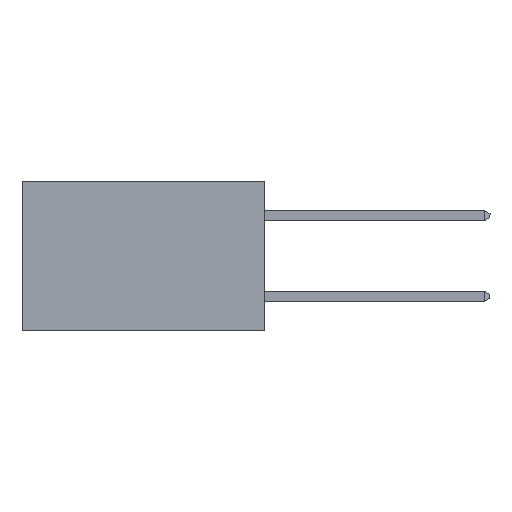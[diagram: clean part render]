
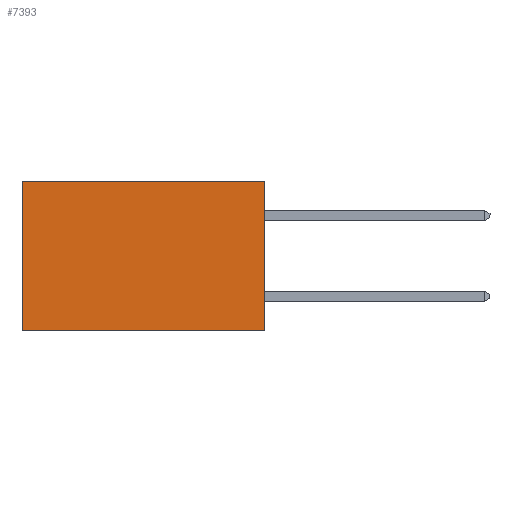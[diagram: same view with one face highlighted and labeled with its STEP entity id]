
A CAD part, left-side view. The second image highlights one B-rep face of the part: STEP entity #7393.
In plain terms, the highlighted planar face has unit normal (-1, 0, 0).
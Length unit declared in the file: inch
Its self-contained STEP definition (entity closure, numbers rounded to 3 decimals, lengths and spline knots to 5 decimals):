
#62 = EDGE_CURVE ( 'NONE', #2784, #5578, #5991, .T. ) ;
#104 = AXIS2_PLACEMENT_3D ( 'NONE', #4249, #1462, #4783 ) ;
#379 = CARTESIAN_POINT ( 'NONE',  ( 0.2615, 0.6, 0. ) ) ;
#814 = CARTESIAN_POINT ( 'NONE',  ( 0.2615, 0.6, -0.37 ) ) ;
#951 = LINE ( 'NONE', #814, #2336 ) ;
#1017 = CARTESIAN_POINT ( 'NONE',  ( 0.2615, 0., -0.37 ) ) ;
#1462 = DIRECTION ( 'NONE',  ( 1., 0., 0. ) ) ;
#1839 = CARTESIAN_POINT ( 'NONE',  ( 0.2615, 0., -0.37 ) ) ;
#1930 = ORIENTED_EDGE ( 'NONE', *, *, #62, .T. ) ;
#2051 = VECTOR ( 'NONE', #7699, 39.37008 ) ;
#2281 = CARTESIAN_POINT ( 'NONE',  ( 0.2615, 0.6, -0.37 ) ) ;
#2336 = VECTOR ( 'NONE', #2877, 39.37008 ) ;
#2393 = CARTESIAN_POINT ( 'NONE',  ( 0.2615, 0., -0.37 ) ) ;
#2560 = VERTEX_POINT ( 'NONE', #2281 ) ;
#2784 = VERTEX_POINT ( 'NONE', #4747 ) ;
#2877 = DIRECTION ( 'NONE',  ( 0., 0., -1. ) ) ;
#2978 = EDGE_CURVE ( 'NONE', #5056, #2560, #4035, .T. ) ;
#3177 = DIRECTION ( 'NONE',  ( 0., 1., 0. ) ) ;
#4035 = LINE ( 'NONE', #1839, #4400 ) ;
#4249 = CARTESIAN_POINT ( 'NONE',  ( 0.2615, 0., -0.37 ) ) ;
#4400 = VECTOR ( 'NONE', #3177, 39.37008 ) ;
#4524 = CARTESIAN_POINT ( 'NONE',  ( 0.2615, 0., 0. ) ) ;
#4747 = CARTESIAN_POINT ( 'NONE',  ( 0.2615, 0., 0. ) ) ;
#4783 = DIRECTION ( 'NONE',  ( 0., 0., -1. ) ) ;
#4790 = VECTOR ( 'NONE', #7992, 39.37008 ) ;
#4991 = EDGE_CURVE ( 'NONE', #2784, #5056, #8448, .T. ) ;
#5056 = VERTEX_POINT ( 'NONE', #2393 ) ;
#5461 = PLANE ( 'NONE',  #104 ) ;
#5578 = VERTEX_POINT ( 'NONE', #379 ) ;
#5921 = EDGE_CURVE ( 'NONE', #5578, #2560, #951, .T. ) ;
#5991 = LINE ( 'NONE', #4524, #4790 ) ;
#6334 = EDGE_LOOP ( 'NONE', ( #6411, #8238, #7669, #1930 ) ) ;
#6411 = ORIENTED_EDGE ( 'NONE', *, *, #5921, .T. ) ;
#7393 = ADVANCED_FACE ( 'NONE', ( #7571 ), #5461, .F. ) ;
#7571 = FACE_OUTER_BOUND ( 'NONE', #6334, .T. ) ;
#7669 = ORIENTED_EDGE ( 'NONE', *, *, #4991, .F. ) ;
#7699 = DIRECTION ( 'NONE',  ( 0., 0., -1. ) ) ;
#7992 = DIRECTION ( 'NONE',  ( 0., 1., 0. ) ) ;
#8238 = ORIENTED_EDGE ( 'NONE', *, *, #2978, .F. ) ;
#8448 = LINE ( 'NONE', #1017, #2051 ) ;
